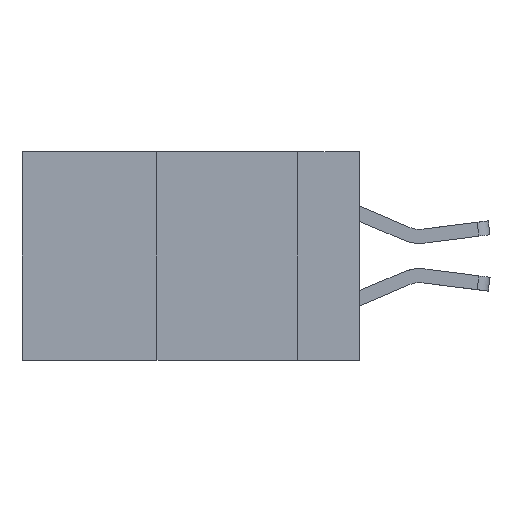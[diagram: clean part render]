
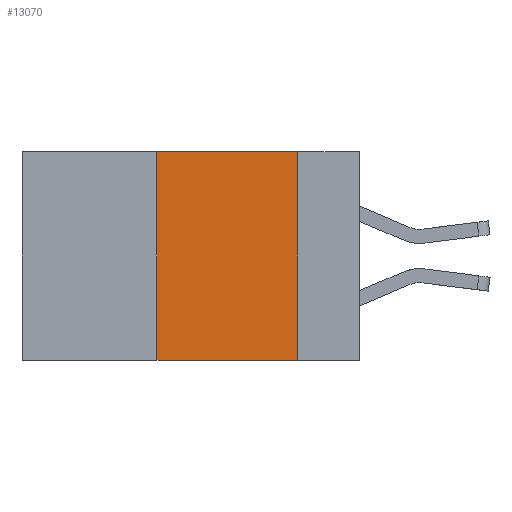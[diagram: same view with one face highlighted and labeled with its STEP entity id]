
A CAD part, left-side view. The second image highlights one B-rep face of the part: STEP entity #13070.
In plain terms, the highlighted planar face has unit normal (-1, 0, 0).
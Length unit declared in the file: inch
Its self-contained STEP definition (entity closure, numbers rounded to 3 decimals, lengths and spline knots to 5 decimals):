
#243 = DIRECTION ( 'NONE',  ( 1., 0., 0. ) ) ;
#563 = CARTESIAN_POINT ( 'NONE',  ( 0., 0.6, -0.37 ) ) ;
#1628 = CARTESIAN_POINT ( 'NONE',  ( 0., 0.36, 0. ) ) ;
#1702 = CARTESIAN_POINT ( 'NONE',  ( 0., 0.11, 0. ) ) ;
#2215 = FACE_OUTER_BOUND ( 'NONE', #4904, .T. ) ;
#2387 = LINE ( 'NONE', #563, #8183 ) ;
#3082 = CARTESIAN_POINT ( 'NONE',  ( 0., 0.6, 0. ) ) ;
#4343 = DIRECTION ( 'NONE',  ( 0., -1., 0. ) ) ;
#4904 = EDGE_LOOP ( 'NONE', ( #10196, #12817, #8441, #7634 ) ) ;
#5208 = VERTEX_POINT ( 'NONE', #13284 ) ;
#5569 = VERTEX_POINT ( 'NONE', #1628 ) ;
#5688 = CARTESIAN_POINT ( 'NONE',  ( 0., 0.36, 0. ) ) ;
#5848 = VECTOR ( 'NONE', #4343, 39.37008 ) ;
#6313 = LINE ( 'NONE', #5688, #8817 ) ;
#6909 = LINE ( 'NONE', #1702, #12189 ) ;
#7367 = CARTESIAN_POINT ( 'NONE',  ( 0., 0.6, 0. ) ) ;
#7634 = ORIENTED_EDGE ( 'NONE', *, *, #13688, .T. ) ;
#8183 = VECTOR ( 'NONE', #10811, 39.37008 ) ;
#8435 = DIRECTION ( 'NONE',  ( 0., 0., -1. ) ) ;
#8441 = ORIENTED_EDGE ( 'NONE', *, *, #14454, .F. ) ;
#8611 = DIRECTION ( 'NONE',  ( 0., 0., -1. ) ) ;
#8762 = EDGE_CURVE ( 'NONE', #9040, #5208, #6909, .T. ) ;
#8817 = VECTOR ( 'NONE', #12055, 39.37008 ) ;
#9040 = VERTEX_POINT ( 'NONE', #13095 ) ;
#9591 = EDGE_CURVE ( 'NONE', #5569, #9040, #14273, .T. ) ;
#10196 = ORIENTED_EDGE ( 'NONE', *, *, #8762, .F. ) ;
#10733 = VERTEX_POINT ( 'NONE', #11749 ) ;
#10811 = DIRECTION ( 'NONE',  ( 0., -1., 0. ) ) ;
#11260 = AXIS2_PLACEMENT_3D ( 'NONE', #7367, #243, #8435 ) ;
#11749 = CARTESIAN_POINT ( 'NONE',  ( 0., 0.36, -0.37 ) ) ;
#12055 = DIRECTION ( 'NONE',  ( 0., 0., 1. ) ) ;
#12189 = VECTOR ( 'NONE', #8611, 39.37008 ) ;
#12817 = ORIENTED_EDGE ( 'NONE', *, *, #9591, .F. ) ;
#13070 = ADVANCED_FACE ( 'NONE', ( #2215 ), #13668, .F. ) ;
#13095 = CARTESIAN_POINT ( 'NONE',  ( 0., 0.11, 0. ) ) ;
#13284 = CARTESIAN_POINT ( 'NONE',  ( 0., 0.11, -0.37 ) ) ;
#13668 = PLANE ( 'NONE',  #11260 ) ;
#13688 = EDGE_CURVE ( 'NONE', #10733, #5208, #2387, .T. ) ;
#14273 = LINE ( 'NONE', #3082, #5848 ) ;
#14454 = EDGE_CURVE ( 'NONE', #10733, #5569, #6313, .T. ) ;
